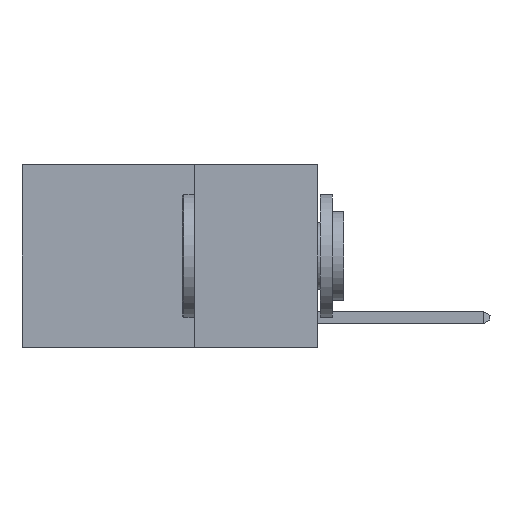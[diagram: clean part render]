
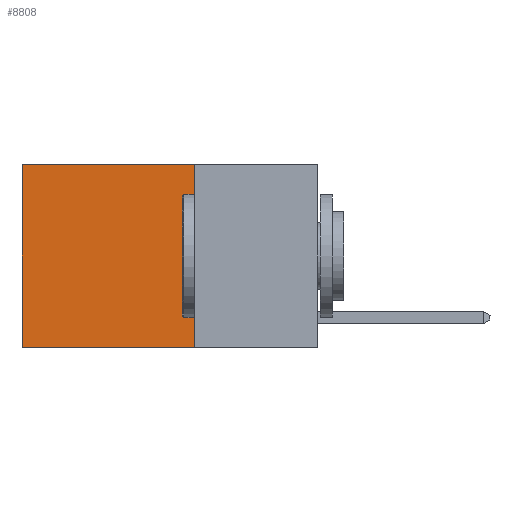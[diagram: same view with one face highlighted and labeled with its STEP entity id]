
A CAD part, left-side view. The second image highlights one B-rep face of the part: STEP entity #8808.
In plain terms, the highlighted planar face has unit normal (-1, 0, 0).
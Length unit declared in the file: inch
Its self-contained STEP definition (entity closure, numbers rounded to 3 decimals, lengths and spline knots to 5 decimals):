
#67 = DIRECTION ( 'NONE',  ( 0., 1., 0. ) ) ;
#376 = EDGE_CURVE ( 'NONE', #5293, #15177, #7078, .T. ) ;
#856 = DIRECTION ( 'NONE',  ( 0., 0., -1. ) ) ;
#2286 = CARTESIAN_POINT ( 'NONE',  ( 0.2625, 0.6, -0.37 ) ) ;
#2571 = VERTEX_POINT ( 'NONE', #16373 ) ;
#5293 = VERTEX_POINT ( 'NONE', #12737 ) ;
#6818 = PLANE ( 'NONE',  #7120 ) ;
#6926 = VECTOR ( 'NONE', #856, 39.37008 ) ;
#6959 = DIRECTION ( 'NONE',  ( 0., 0., -1. ) ) ;
#7078 = LINE ( 'NONE', #20619, #12661 ) ;
#7120 = AXIS2_PLACEMENT_3D ( 'NONE', #20793, #11013, #6959 ) ;
#7535 = ORIENTED_EDGE ( 'NONE', *, *, #21365, .T. ) ;
#8592 = CARTESIAN_POINT ( 'NONE',  ( 0.2625, 0.6, 0. ) ) ;
#8808 = ADVANCED_FACE ( 'NONE', ( #13414 ), #6818, .F. ) ;
#10769 = DIRECTION ( 'NONE',  ( 0., 0., -1. ) ) ;
#10819 = VERTEX_POINT ( 'NONE', #8592 ) ;
#11013 = DIRECTION ( 'NONE',  ( 1., 0., 0. ) ) ;
#11444 = ORIENTED_EDGE ( 'NONE', *, *, #22821, .T. ) ;
#11496 = EDGE_LOOP ( 'NONE', ( #7535, #12328, #27623, #11444 ) ) ;
#11880 = VECTOR ( 'NONE', #10769, 39.37008 ) ;
#12328 = ORIENTED_EDGE ( 'NONE', *, *, #376, .F. ) ;
#12661 = VECTOR ( 'NONE', #67, 39.37008 ) ;
#12737 = CARTESIAN_POINT ( 'NONE',  ( 0.2625, 0.25, -0.37 ) ) ;
#13023 = EDGE_CURVE ( 'NONE', #2571, #5293, #29067, .T. ) ;
#13414 = FACE_OUTER_BOUND ( 'NONE', #11496, .T. ) ;
#13480 = CARTESIAN_POINT ( 'NONE',  ( 0.2625, 0.25, 0. ) ) ;
#15177 = VERTEX_POINT ( 'NONE', #2286 ) ;
#15636 = VECTOR ( 'NONE', #17044, 39.37008 ) ;
#16373 = CARTESIAN_POINT ( 'NONE',  ( 0.2625, 0.25, 0. ) ) ;
#17044 = DIRECTION ( 'NONE',  ( 0., 1., 0. ) ) ;
#20619 = CARTESIAN_POINT ( 'NONE',  ( 0.2625, 0.25, -0.37 ) ) ;
#20793 = CARTESIAN_POINT ( 'NONE',  ( 0.2625, 0.25, 0. ) ) ;
#21365 = EDGE_CURVE ( 'NONE', #10819, #15177, #26051, .T. ) ;
#21560 = CARTESIAN_POINT ( 'NONE',  ( 0.2625, 0.6, 0. ) ) ;
#22821 = EDGE_CURVE ( 'NONE', #2571, #10819, #26504, .T. ) ;
#26051 = LINE ( 'NONE', #21560, #6926 ) ;
#26504 = LINE ( 'NONE', #28440, #15636 ) ;
#27623 = ORIENTED_EDGE ( 'NONE', *, *, #13023, .F. ) ;
#28440 = CARTESIAN_POINT ( 'NONE',  ( 0.2625, 0.25, 0. ) ) ;
#29067 = LINE ( 'NONE', #13480, #11880 ) ;
